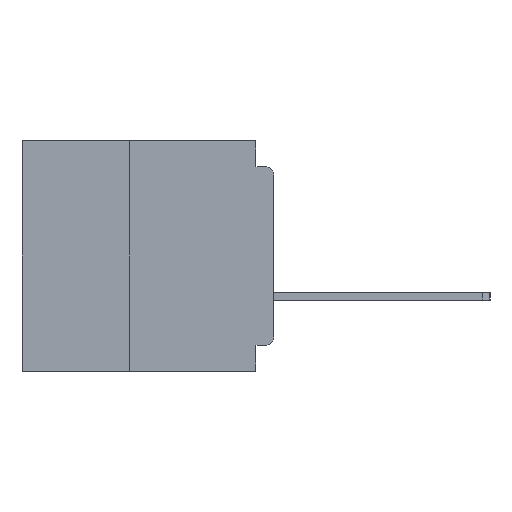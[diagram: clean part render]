
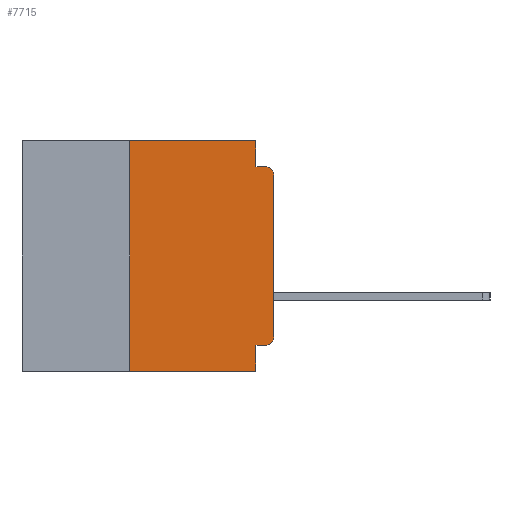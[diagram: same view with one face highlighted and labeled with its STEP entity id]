
A CAD part, left-side view. The second image highlights one B-rep face of the part: STEP entity #7715.
In plain terms, the highlighted planar face has unit normal (-1, 0, 0).
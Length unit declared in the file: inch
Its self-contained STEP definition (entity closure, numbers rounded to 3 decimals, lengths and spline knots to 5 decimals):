
#182 = EDGE_CURVE ( 'NONE', #26639, #33181, #27867, .T. ) ;
#830 = CARTESIAN_POINT ( 'NONE',  ( 0., 0.25, -0.4 ) ) ;
#949 = AXIS2_PLACEMENT_3D ( 'NONE', #34399, #5164, #39265 ) ;
#1019 = ORIENTED_EDGE ( 'NONE', *, *, #182, .F. ) ;
#1095 = VECTOR ( 'NONE', #10611, 39.37008 ) ;
#2342 = DIRECTION ( 'NONE',  ( 0., -1., 0. ) ) ;
#4947 = DIRECTION ( 'NONE',  ( -1., 0., 0. ) ) ;
#5164 = DIRECTION ( 'NONE',  ( -1., 0., 0. ) ) ;
#5972 = CARTESIAN_POINT ( 'NONE',  ( 0., 0.437, -0.4 ) ) ;
#6707 = VERTEX_POINT ( 'NONE', #24609 ) ;
#7087 = EDGE_LOOP ( 'NONE', ( #14084, #54529, #1019, #18631, #61184, #42699, #14790, #48526, #56430, #15367 ) ) ;
#7715 = ADVANCED_FACE ( 'NONE', ( #39108 ), #10622, .F. ) ;
#8313 = DIRECTION ( 'NONE',  ( 0., 0., -1. ) ) ;
#9707 = CARTESIAN_POINT ( 'NONE',  ( 0., 0., -0.06 ) ) ;
#9796 = CARTESIAN_POINT ( 'NONE',  ( 0., 0.25, -0.4 ) ) ;
#10611 = DIRECTION ( 'NONE',  ( 0., -1., 0. ) ) ;
#10622 = PLANE ( 'NONE',  #19177 ) ;
#10834 = CARTESIAN_POINT ( 'NONE',  ( 0., 0., -0.355 ) ) ;
#11387 = VECTOR ( 'NONE', #44969, 39.37008 ) ;
#11508 = VECTOR ( 'NONE', #19298, 39.37008 ) ;
#12055 = CIRCLE ( 'NONE', #949, 0.015 ) ;
#12791 = CIRCLE ( 'NONE', #34748, 0.015 ) ;
#14084 = ORIENTED_EDGE ( 'NONE', *, *, #29524, .T. ) ;
#14790 = ORIENTED_EDGE ( 'NONE', *, *, #19174, .T. ) ;
#15367 = ORIENTED_EDGE ( 'NONE', *, *, #33248, .T. ) ;
#15584 = DIRECTION ( 'NONE',  ( 1., 0., 0. ) ) ;
#16475 = VECTOR ( 'NONE', #2342, 39.37008 ) ;
#18371 = LINE ( 'NONE', #47325, #41157 ) ;
#18631 = ORIENTED_EDGE ( 'NONE', *, *, #54270, .F. ) ;
#19174 = EDGE_CURVE ( 'NONE', #24493, #55701, #48731, .T. ) ;
#19177 = AXIS2_PLACEMENT_3D ( 'NONE', #30026, #15584, #49568 ) ;
#19298 = DIRECTION ( 'NONE',  ( 0., 0., -1. ) ) ;
#20292 = VERTEX_POINT ( 'NONE', #9707 ) ;
#21477 = CARTESIAN_POINT ( 'NONE',  ( 0., 0.031, -0.4 ) ) ;
#21975 = LINE ( 'NONE', #9796, #47859 ) ;
#22180 = CARTESIAN_POINT ( 'NONE',  ( 0., 0.015, -0.355 ) ) ;
#23268 = CARTESIAN_POINT ( 'NONE',  ( 0., 0., 0. ) ) ;
#23292 = CARTESIAN_POINT ( 'NONE',  ( 0., 0., -0.34 ) ) ;
#24493 = VERTEX_POINT ( 'NONE', #830 ) ;
#24609 = CARTESIAN_POINT ( 'NONE',  ( 0., 0.031, -0.355 ) ) ;
#25604 = CARTESIAN_POINT ( 'NONE',  ( 0., 0.25, 0. ) ) ;
#25810 = EDGE_CURVE ( 'NONE', #37491, #35765, #28665, .T. ) ;
#26001 = LINE ( 'NONE', #29058, #11508 ) ;
#26639 = VERTEX_POINT ( 'NONE', #55871 ) ;
#27867 = LINE ( 'NONE', #51212, #16475 ) ;
#28665 = LINE ( 'NONE', #39536, #1095 ) ;
#29058 = CARTESIAN_POINT ( 'NONE',  ( 0., 0.031, 0. ) ) ;
#29491 = EDGE_CURVE ( 'NONE', #6707, #55701, #18371, .T. ) ;
#29524 = EDGE_CURVE ( 'NONE', #43992, #20292, #39622, .T. ) ;
#30026 = CARTESIAN_POINT ( 'NONE',  ( 0., 0.437, 0. ) ) ;
#30295 = CARTESIAN_POINT ( 'NONE',  ( 0., 0.031, 0. ) ) ;
#33181 = VERTEX_POINT ( 'NONE', #38651 ) ;
#33248 = EDGE_CURVE ( 'NONE', #39047, #43992, #12055, .T. ) ;
#34182 = CARTESIAN_POINT ( 'NONE',  ( 0., 0.015, -0.06 ) ) ;
#34399 = CARTESIAN_POINT ( 'NONE',  ( 0., 0.015, -0.34 ) ) ;
#34748 = AXIS2_PLACEMENT_3D ( 'NONE', #34182, #4947, #39040 ) ;
#35765 = VERTEX_POINT ( 'NONE', #30295 ) ;
#37491 = VERTEX_POINT ( 'NONE', #25604 ) ;
#38572 = EDGE_CURVE ( 'NONE', #20292, #33181, #12791, .T. ) ;
#38651 = CARTESIAN_POINT ( 'NONE',  ( 0., 0.015, -0.045 ) ) ;
#38948 = DIRECTION ( 'NONE',  ( 0., 0., 1. ) ) ;
#39040 = DIRECTION ( 'NONE',  ( 0., 0., -1. ) ) ;
#39047 = VERTEX_POINT ( 'NONE', #22180 ) ;
#39108 = FACE_OUTER_BOUND ( 'NONE', #7087, .T. ) ;
#39265 = DIRECTION ( 'NONE',  ( 0., 0., -1. ) ) ;
#39536 = CARTESIAN_POINT ( 'NONE',  ( 0., 0.437, 0. ) ) ;
#39622 = LINE ( 'NONE', #23268, #52600 ) ;
#41157 = VECTOR ( 'NONE', #8313, 39.37008 ) ;
#42699 = ORIENTED_EDGE ( 'NONE', *, *, #58929, .F. ) ;
#43992 = VERTEX_POINT ( 'NONE', #23292 ) ;
#44969 = DIRECTION ( 'NONE',  ( 0., -1., 0. ) ) ;
#47325 = CARTESIAN_POINT ( 'NONE',  ( 0., 0.031, -0.4 ) ) ;
#47859 = VECTOR ( 'NONE', #38948, 39.37008 ) ;
#48526 = ORIENTED_EDGE ( 'NONE', *, *, #29491, .F. ) ;
#48731 = LINE ( 'NONE', #5972, #11387 ) ;
#49568 = DIRECTION ( 'NONE',  ( 0., 0., -1. ) ) ;
#49755 = VECTOR ( 'NONE', #49783, 39.37008 ) ;
#49783 = DIRECTION ( 'NONE',  ( 0., 1., 0. ) ) ;
#51212 = CARTESIAN_POINT ( 'NONE',  ( 0., 0., -0.045 ) ) ;
#51304 = LINE ( 'NONE', #10834, #49755 ) ;
#51732 = EDGE_CURVE ( 'NONE', #39047, #6707, #51304, .T. ) ;
#52386 = DIRECTION ( 'NONE',  ( 0., 0., 1. ) ) ;
#52600 = VECTOR ( 'NONE', #52386, 39.37008 ) ;
#54270 = EDGE_CURVE ( 'NONE', #35765, #26639, #26001, .T. ) ;
#54529 = ORIENTED_EDGE ( 'NONE', *, *, #38572, .T. ) ;
#55701 = VERTEX_POINT ( 'NONE', #21477 ) ;
#55871 = CARTESIAN_POINT ( 'NONE',  ( 0., 0.031, -0.045 ) ) ;
#56430 = ORIENTED_EDGE ( 'NONE', *, *, #51732, .F. ) ;
#58929 = EDGE_CURVE ( 'NONE', #24493, #37491, #21975, .T. ) ;
#61184 = ORIENTED_EDGE ( 'NONE', *, *, #25810, .F. ) ;
